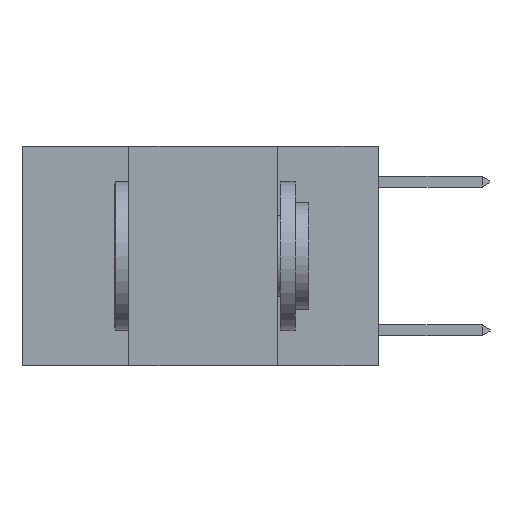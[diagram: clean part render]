
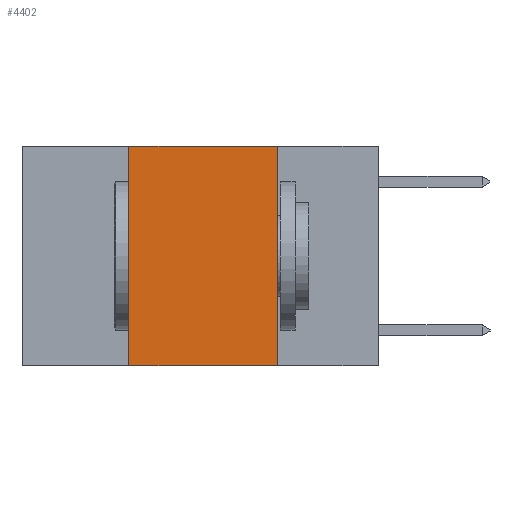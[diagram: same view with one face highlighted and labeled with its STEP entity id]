
A CAD part, left-side view. The second image highlights one B-rep face of the part: STEP entity #4402.
In plain terms, the highlighted planar face has unit normal (-1, 0, 0).
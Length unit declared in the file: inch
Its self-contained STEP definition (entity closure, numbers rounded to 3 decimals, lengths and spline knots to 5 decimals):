
#73 = ORIENTED_EDGE ( 'NONE', *, *, #4858, .F. ) ;
#546 = EDGE_CURVE ( 'NONE', #2110, #1226, #5378, .T. ) ;
#796 = VECTOR ( 'NONE', #1779, 39.37008 ) ;
#868 = LINE ( 'NONE', #5329, #4523 ) ;
#1226 = VERTEX_POINT ( 'NONE', #6113 ) ;
#1239 = DIRECTION ( 'NONE',  ( 0., 0., -1. ) ) ;
#1495 = VECTOR ( 'NONE', #1239, 39.37008 ) ;
#1779 = DIRECTION ( 'NONE',  ( 0., -1., 0. ) ) ;
#2110 = VERTEX_POINT ( 'NONE', #4253 ) ;
#2464 = EDGE_CURVE ( 'NONE', #9217, #1226, #868, .T. ) ;
#2570 = DIRECTION ( 'NONE',  ( 1., 0., 0. ) ) ;
#3327 = LINE ( 'NONE', #8282, #7237 ) ;
#3857 = DIRECTION ( 'NONE',  ( 0., 0., 1. ) ) ;
#4162 = ORIENTED_EDGE ( 'NONE', *, *, #6776, .F. ) ;
#4253 = CARTESIAN_POINT ( 'NONE',  ( 0., 0.17, 0. ) ) ;
#4402 = ADVANCED_FACE ( 'NONE', ( #7244 ), #6943, .F. ) ;
#4523 = VECTOR ( 'NONE', #7572, 39.37008 ) ;
#4540 = AXIS2_PLACEMENT_3D ( 'NONE', #6193, #2570, #7695 ) ;
#4673 = LINE ( 'NONE', #9118, #796 ) ;
#4858 = EDGE_CURVE ( 'NONE', #9217, #8562, #3327, .T. ) ;
#4913 = CARTESIAN_POINT ( 'NONE',  ( 0., 0.42, -0.37 ) ) ;
#5329 = CARTESIAN_POINT ( 'NONE',  ( 0., 0.6, -0.37 ) ) ;
#5378 = LINE ( 'NONE', #5570, #1495 ) ;
#5570 = CARTESIAN_POINT ( 'NONE',  ( 0., 0.17, 0. ) ) ;
#6113 = CARTESIAN_POINT ( 'NONE',  ( 0., 0.17, -0.37 ) ) ;
#6193 = CARTESIAN_POINT ( 'NONE',  ( 0., 0.6, 0. ) ) ;
#6776 = EDGE_CURVE ( 'NONE', #8562, #2110, #4673, .T. ) ;
#6943 = PLANE ( 'NONE',  #4540 ) ;
#7237 = VECTOR ( 'NONE', #3857, 39.37008 ) ;
#7244 = FACE_OUTER_BOUND ( 'NONE', #7419, .T. ) ;
#7419 = EDGE_LOOP ( 'NONE', ( #8401, #4162, #73, #8690 ) ) ;
#7572 = DIRECTION ( 'NONE',  ( 0., -1., 0. ) ) ;
#7695 = DIRECTION ( 'NONE',  ( 0., 0., -1. ) ) ;
#8282 = CARTESIAN_POINT ( 'NONE',  ( 0., 0.42, 0. ) ) ;
#8401 = ORIENTED_EDGE ( 'NONE', *, *, #546, .F. ) ;
#8562 = VERTEX_POINT ( 'NONE', #9364 ) ;
#8690 = ORIENTED_EDGE ( 'NONE', *, *, #2464, .T. ) ;
#9118 = CARTESIAN_POINT ( 'NONE',  ( 0., 0.6, 0. ) ) ;
#9217 = VERTEX_POINT ( 'NONE', #4913 ) ;
#9364 = CARTESIAN_POINT ( 'NONE',  ( 0., 0.42, 0. ) ) ;
